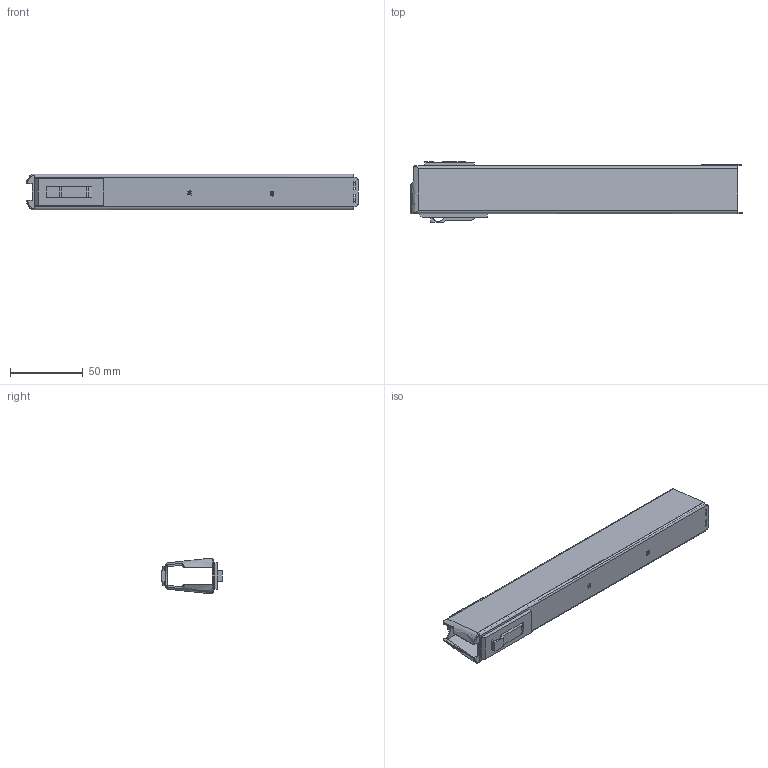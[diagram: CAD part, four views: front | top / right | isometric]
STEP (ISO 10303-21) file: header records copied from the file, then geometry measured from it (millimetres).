
FILE_DESCRIPTION (( 'STEP AP214' ), '1' );
FILE_NAME ('m45B magasin - 015.STEP', '2020-10-09T21:06:10', ( '' ), ( '' ), 'SwSTEP 2.0', 'SolidWorks 2020', '' );
FILE_SCHEMA (( 'AUTOMOTIVE_DESIGN' ));
Length unit declared in the file: millimetre
Products named in the file (1): m45B magasin - 015
Bounding box: 228.73 x 42 x 24.55 mm (x, y, z)
Volume: 26995.4 mm3; surface area: 47819.4 mm2
Topology: 2 solids, 2 shells, 177 faces, 492 edges, 324 vertices
Faces by surface type: plane 106, bspline 51, cylinder 16, torus 4
Entity records: 8136 total; most frequent: CARTESIAN_POINT 3931, ORIENTED_EDGE 984, DIRECTION 634, EDGE_CURVE 492, VERTEX_POINT 324, LINE 314, VECTOR 314, EDGE_LOOP 192
